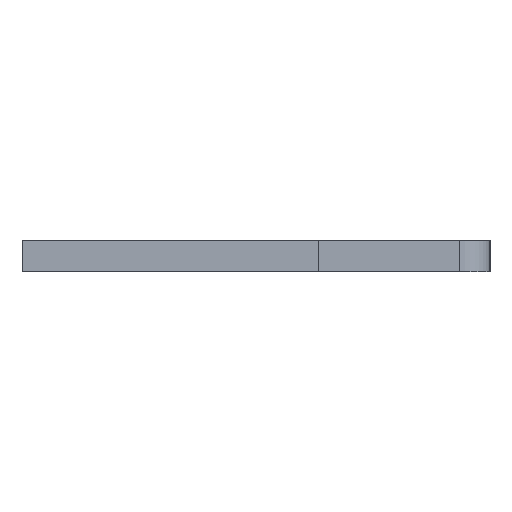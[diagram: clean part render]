
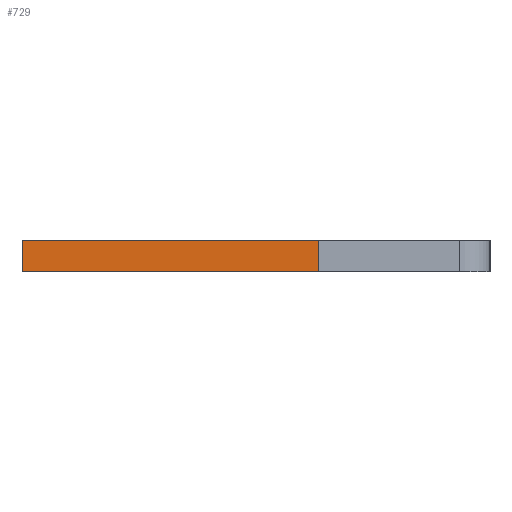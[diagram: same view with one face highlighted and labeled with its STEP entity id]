
A CAD part, left-side view. The second image highlights one B-rep face of the part: STEP entity #729.
In plain terms, the highlighted face is planar.
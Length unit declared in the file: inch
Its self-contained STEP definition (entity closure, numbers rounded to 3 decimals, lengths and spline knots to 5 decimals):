
#99 = DIRECTION ( 'NONE',  ( 0., 0., 1. ) ) ;
#117 = CARTESIAN_POINT ( 'NONE',  ( 0.01, 0.15, -0.04 ) ) ;
#279 = CARTESIAN_POINT ( 'NONE',  ( 0.01, -0.04, -0.04 ) ) ;
#316 = EDGE_CURVE ( 'NONE', #999, #2489, #1084, .T. ) ;
#339 = CARTESIAN_POINT ( 'NONE',  ( -0.01, 0.15, -0.04 ) ) ;
#570 = VECTOR ( 'NONE', #1691, 39.37008 ) ;
#729 = ADVANCED_FACE ( 'NONE', ( #1340 ), #864, .F. ) ;
#829 = EDGE_CURVE ( 'NONE', #1751, #999, #1193, .T. ) ;
#847 = ORIENTED_EDGE ( 'NONE', *, *, #1334, .T. ) ;
#864 = PLANE ( 'NONE',  #1293 ) ;
#907 = DIRECTION ( 'NONE',  ( 1., 0., 0. ) ) ;
#988 = CARTESIAN_POINT ( 'NONE',  ( 0.01, 0.15, -0.04 ) ) ;
#999 = VERTEX_POINT ( 'NONE', #1746 ) ;
#1024 = EDGE_LOOP ( 'NONE', ( #2215, #1484, #1904, #847 ) ) ;
#1026 = DIRECTION ( 'NONE',  ( -1., 0., 0. ) ) ;
#1084 = LINE ( 'NONE', #988, #2273 ) ;
#1159 = CARTESIAN_POINT ( 'NONE',  ( -0.01, -0.04, -0.04 ) ) ;
#1193 = LINE ( 'NONE', #117, #2055 ) ;
#1293 = AXIS2_PLACEMENT_3D ( 'NONE', #2450, #99, #907 ) ;
#1334 = EDGE_CURVE ( 'NONE', #1751, #2218, #1405, .T. ) ;
#1340 = FACE_OUTER_BOUND ( 'NONE', #1024, .T. ) ;
#1405 = LINE ( 'NONE', #279, #2142 ) ;
#1484 = ORIENTED_EDGE ( 'NONE', *, *, #316, .F. ) ;
#1491 = LINE ( 'NONE', #339, #570 ) ;
#1503 = CARTESIAN_POINT ( 'NONE',  ( 0.01, -0.04, -0.04 ) ) ;
#1522 = DIRECTION ( 'NONE',  ( 0., 1., 0. ) ) ;
#1676 = EDGE_CURVE ( 'NONE', #2218, #2489, #1491, .T. ) ;
#1691 = DIRECTION ( 'NONE',  ( 0., 1., 0. ) ) ;
#1746 = CARTESIAN_POINT ( 'NONE',  ( 0.01, 0.15, -0.04 ) ) ;
#1751 = VERTEX_POINT ( 'NONE', #1503 ) ;
#1904 = ORIENTED_EDGE ( 'NONE', *, *, #829, .F. ) ;
#1963 = CARTESIAN_POINT ( 'NONE',  ( -0.01, 0.15, -0.04 ) ) ;
#2055 = VECTOR ( 'NONE', #1522, 39.37008 ) ;
#2142 = VECTOR ( 'NONE', #1026, 39.37008 ) ;
#2179 = DIRECTION ( 'NONE',  ( -1., 0., 0. ) ) ;
#2215 = ORIENTED_EDGE ( 'NONE', *, *, #1676, .T. ) ;
#2218 = VERTEX_POINT ( 'NONE', #1159 ) ;
#2273 = VECTOR ( 'NONE', #2179, 39.37008 ) ;
#2450 = CARTESIAN_POINT ( 'NONE',  ( 0.01, 0.15, -0.04 ) ) ;
#2489 = VERTEX_POINT ( 'NONE', #1963 ) ;
